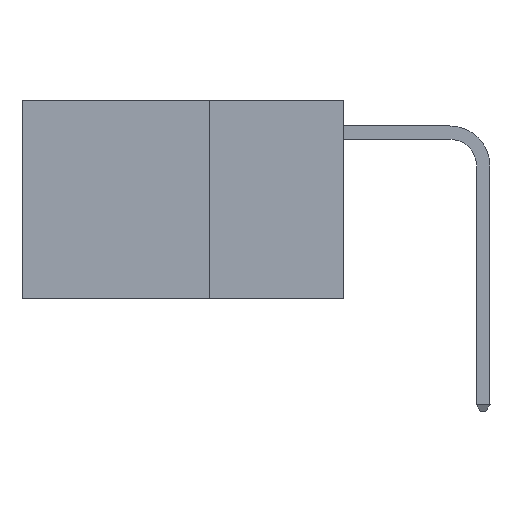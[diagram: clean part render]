
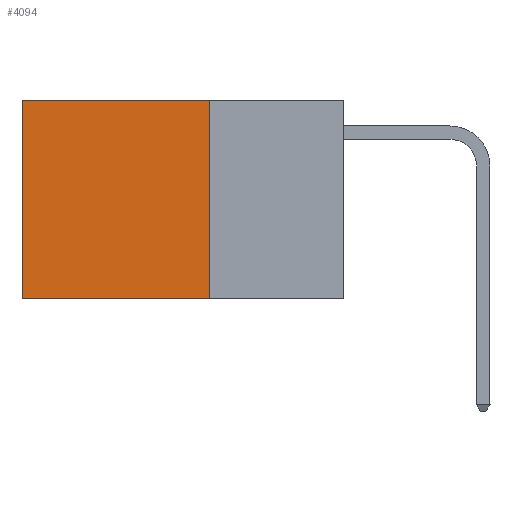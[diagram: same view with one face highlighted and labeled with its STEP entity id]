
A CAD part, left-side view. The second image highlights one B-rep face of the part: STEP entity #4094.
In plain terms, the highlighted planar face has unit normal (-1, 0, 0).
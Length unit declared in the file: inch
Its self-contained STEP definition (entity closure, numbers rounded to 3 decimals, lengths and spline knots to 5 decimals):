
#176 = VERTEX_POINT ( 'NONE', #1040 ) ;
#357 = PLANE ( 'NONE',  #2667 ) ;
#414 = CARTESIAN_POINT ( 'NONE',  ( 0.2625, 0.25, 0. ) ) ;
#475 = EDGE_CURVE ( 'NONE', #8114, #4492, #3627, .T. ) ;
#880 = VECTOR ( 'NONE', #3554, 39.37008 ) ;
#1040 = CARTESIAN_POINT ( 'NONE',  ( 0.2625, 0.6, 0. ) ) ;
#1415 = CARTESIAN_POINT ( 'NONE',  ( 0.2625, 0.6, 0. ) ) ;
#1518 = CARTESIAN_POINT ( 'NONE',  ( 0.2625, 0.25, 0. ) ) ;
#1755 = DIRECTION ( 'NONE',  ( 0., 0., -1. ) ) ;
#1994 = ORIENTED_EDGE ( 'NONE', *, *, #3667, .T. ) ;
#2250 = VECTOR ( 'NONE', #6445, 39.37008 ) ;
#2527 = CARTESIAN_POINT ( 'NONE',  ( 0.2625, 0.25, 0. ) ) ;
#2667 = AXIS2_PLACEMENT_3D ( 'NONE', #5035, #5636, #1755 ) ;
#2761 = EDGE_LOOP ( 'NONE', ( #4877, #3374, #5276, #1994 ) ) ;
#3113 = CARTESIAN_POINT ( 'NONE',  ( 0.2625, 0.25, -0.37 ) ) ;
#3208 = DIRECTION ( 'NONE',  ( 0., 1., 0. ) ) ;
#3374 = ORIENTED_EDGE ( 'NONE', *, *, #475, .F. ) ;
#3554 = DIRECTION ( 'NONE',  ( 0., 0., -1. ) ) ;
#3627 = LINE ( 'NONE', #3113, #2250 ) ;
#3667 = EDGE_CURVE ( 'NONE', #4720, #176, #5155, .T. ) ;
#4094 = ADVANCED_FACE ( 'NONE', ( #6470 ), #357, .F. ) ;
#4492 = VERTEX_POINT ( 'NONE', #6581 ) ;
#4552 = EDGE_CURVE ( 'NONE', #4720, #8114, #6099, .T. ) ;
#4720 = VERTEX_POINT ( 'NONE', #414 ) ;
#4877 = ORIENTED_EDGE ( 'NONE', *, *, #5119, .T. ) ;
#5035 = CARTESIAN_POINT ( 'NONE',  ( 0.2625, 0.25, 0. ) ) ;
#5119 = EDGE_CURVE ( 'NONE', #176, #4492, #6275, .T. ) ;
#5155 = LINE ( 'NONE', #2527, #8046 ) ;
#5276 = ORIENTED_EDGE ( 'NONE', *, *, #4552, .F. ) ;
#5572 = CARTESIAN_POINT ( 'NONE',  ( 0.2625, 0.25, -0.37 ) ) ;
#5636 = DIRECTION ( 'NONE',  ( 1., 0., 0. ) ) ;
#6090 = VECTOR ( 'NONE', #6550, 39.37008 ) ;
#6099 = LINE ( 'NONE', #1518, #880 ) ;
#6275 = LINE ( 'NONE', #1415, #6090 ) ;
#6445 = DIRECTION ( 'NONE',  ( 0., 1., 0. ) ) ;
#6470 = FACE_OUTER_BOUND ( 'NONE', #2761, .T. ) ;
#6550 = DIRECTION ( 'NONE',  ( 0., 0., -1. ) ) ;
#6581 = CARTESIAN_POINT ( 'NONE',  ( 0.2625, 0.6, -0.37 ) ) ;
#8046 = VECTOR ( 'NONE', #3208, 39.37008 ) ;
#8114 = VERTEX_POINT ( 'NONE', #5572 ) ;
